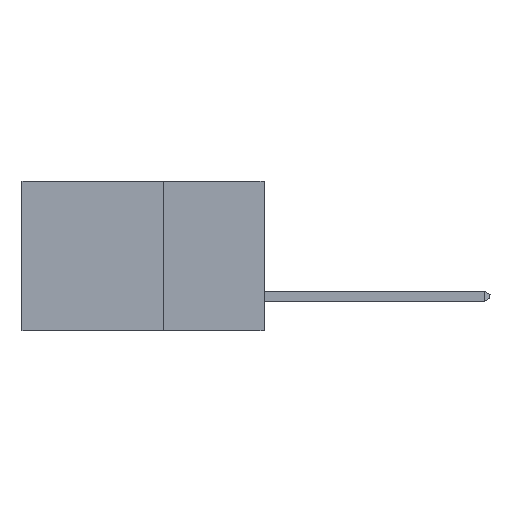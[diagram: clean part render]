
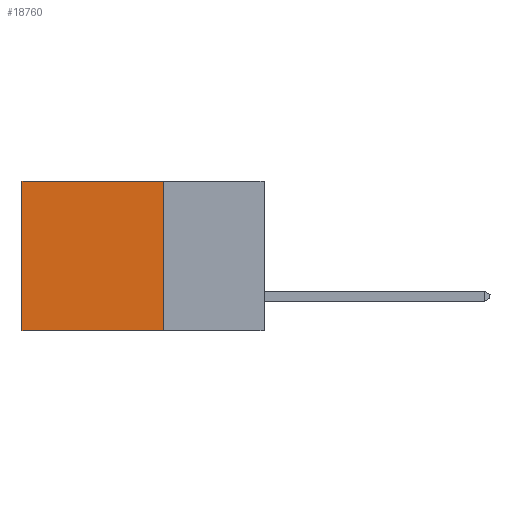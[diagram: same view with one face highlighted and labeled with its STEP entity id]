
A CAD part, left-side view. The second image highlights one B-rep face of the part: STEP entity #18760.
In plain terms, the highlighted planar face has unit normal (-1, 0, 0).
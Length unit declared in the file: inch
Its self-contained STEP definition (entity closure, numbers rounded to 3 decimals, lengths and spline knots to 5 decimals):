
#186 = CARTESIAN_POINT ( 'NONE',  ( 0.2615, 0.6, -0.37 ) ) ;
#302 = LINE ( 'NONE', #9156, #11375 ) ;
#320 = DIRECTION ( 'NONE',  ( 0., 1., 0. ) ) ;
#1610 = VERTEX_POINT ( 'NONE', #4262 ) ;
#1991 = ORIENTED_EDGE ( 'NONE', *, *, #5137, .F. ) ;
#2332 = ORIENTED_EDGE ( 'NONE', *, *, #11023, .F. ) ;
#2798 = EDGE_LOOP ( 'NONE', ( #15839, #2332, #1991, #12064 ) ) ;
#3785 = EDGE_CURVE ( 'NONE', #7871, #1610, #302, .T. ) ;
#4262 = CARTESIAN_POINT ( 'NONE',  ( 0.2615, 0.6, 0. ) ) ;
#4396 = CARTESIAN_POINT ( 'NONE',  ( 0.2615, 0.25, -0.37 ) ) ;
#5083 = VERTEX_POINT ( 'NONE', #9583 ) ;
#5108 = FACE_OUTER_BOUND ( 'NONE', #2798, .T. ) ;
#5137 = EDGE_CURVE ( 'NONE', #7871, #12236, #19873, .T. ) ;
#6234 = VECTOR ( 'NONE', #19557, 39.37008 ) ;
#7681 = CARTESIAN_POINT ( 'NONE',  ( 0.2615, 0.25, -0.37 ) ) ;
#7871 = VERTEX_POINT ( 'NONE', #18882 ) ;
#8728 = LINE ( 'NONE', #20351, #17221 ) ;
#8742 = CARTESIAN_POINT ( 'NONE',  ( 0.2615, 0.25, -0.37 ) ) ;
#9156 = CARTESIAN_POINT ( 'NONE',  ( 0.2615, 0.25, 0. ) ) ;
#9583 = CARTESIAN_POINT ( 'NONE',  ( 0.2615, 0.6, -0.37 ) ) ;
#9819 = DIRECTION ( 'NONE',  ( 0., 0., -1. ) ) ;
#10184 = PLANE ( 'NONE',  #19521 ) ;
#10214 = EDGE_CURVE ( 'NONE', #1610, #5083, #15352, .T. ) ;
#11023 = EDGE_CURVE ( 'NONE', #12236, #5083, #8728, .T. ) ;
#11375 = VECTOR ( 'NONE', #20984, 39.37008 ) ;
#11870 = DIRECTION ( 'NONE',  ( 1., 0., 0. ) ) ;
#12064 = ORIENTED_EDGE ( 'NONE', *, *, #3785, .T. ) ;
#12236 = VERTEX_POINT ( 'NONE', #7681 ) ;
#15352 = LINE ( 'NONE', #186, #16495 ) ;
#15839 = ORIENTED_EDGE ( 'NONE', *, *, #10214, .T. ) ;
#16495 = VECTOR ( 'NONE', #9819, 39.37008 ) ;
#17221 = VECTOR ( 'NONE', #320, 39.37008 ) ;
#18594 = DIRECTION ( 'NONE',  ( 0., 0., -1. ) ) ;
#18760 = ADVANCED_FACE ( 'NONE', ( #5108 ), #10184, .F. ) ;
#18882 = CARTESIAN_POINT ( 'NONE',  ( 0.2615, 0.25, 0. ) ) ;
#19521 = AXIS2_PLACEMENT_3D ( 'NONE', #8742, #11870, #18594 ) ;
#19557 = DIRECTION ( 'NONE',  ( 0., 0., -1. ) ) ;
#19873 = LINE ( 'NONE', #4396, #6234 ) ;
#20351 = CARTESIAN_POINT ( 'NONE',  ( 0.2615, 0.25, -0.37 ) ) ;
#20984 = DIRECTION ( 'NONE',  ( 0., 1., 0. ) ) ;
